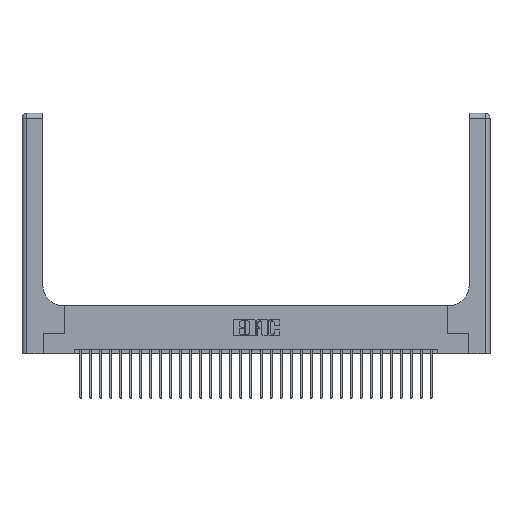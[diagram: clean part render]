
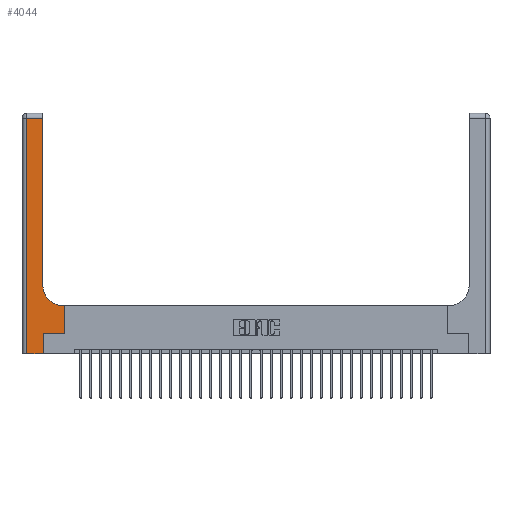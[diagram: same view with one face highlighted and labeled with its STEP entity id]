
A CAD part, top view. The second image highlights one B-rep face of the part: STEP entity #4044.
In plain terms, the highlighted planar face has unit normal (0, 0, 1).
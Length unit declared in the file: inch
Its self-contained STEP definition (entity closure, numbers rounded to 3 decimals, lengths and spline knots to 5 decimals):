
#496 = DIRECTION ( 'NONE',  ( 0., 1., 0. ) ) ;
#600 = VECTOR ( 'NONE', #2270, 39.37008 ) ;
#1074 = EDGE_CURVE ( 'NONE', #3057, #27506, #25607, .T. ) ;
#1107 = LINE ( 'NONE', #29001, #22637 ) ;
#1512 = CARTESIAN_POINT ( 'NONE',  ( 0.528, 0.6, 0.37 ) ) ;
#1595 = VERTEX_POINT ( 'NONE', #16733 ) ;
#1620 = CARTESIAN_POINT ( 'NONE',  ( 0.06, 3., 0.37 ) ) ;
#1677 = CARTESIAN_POINT ( 'NONE',  ( 0.265, 0., 0.37 ) ) ;
#1723 = DIRECTION ( 'NONE',  ( 0., 0., -1. ) ) ;
#1886 = CARTESIAN_POINT ( 'NONE',  ( 0., 3., 0.37 ) ) ;
#2270 = DIRECTION ( 'NONE',  ( 1., 0., 0. ) ) ;
#2606 = VECTOR ( 'NONE', #24935, 39.37008 ) ;
#3057 = VERTEX_POINT ( 'NONE', #15080 ) ;
#3181 = VERTEX_POINT ( 'NONE', #25020 ) ;
#3529 = CARTESIAN_POINT ( 'NONE',  ( 0.26, 0.85, 0.37 ) ) ;
#4044 = ADVANCED_FACE ( 'NONE', ( #29774 ), #22447, .F. ) ;
#4904 = ORIENTED_EDGE ( 'NONE', *, *, #13487, .T. ) ;
#5570 = CARTESIAN_POINT ( 'NONE',  ( 0.06, 2.94, 0.37 ) ) ;
#5603 = AXIS2_PLACEMENT_3D ( 'NONE', #1886, #1723, #27196 ) ;
#5758 = VECTOR ( 'NONE', #496, 39.37008 ) ;
#5967 = VERTEX_POINT ( 'NONE', #1512 ) ;
#6433 = EDGE_CURVE ( 'NONE', #5967, #1595, #26345, .T. ) ;
#7788 = ORIENTED_EDGE ( 'NONE', *, *, #6433, .T. ) ;
#7836 = CARTESIAN_POINT ( 'NONE',  ( 0., 0., 0.37 ) ) ;
#7870 = EDGE_CURVE ( 'NONE', #19559, #3181, #12021, .T. ) ;
#10801 = VERTEX_POINT ( 'NONE', #1677 ) ;
#10849 = CARTESIAN_POINT ( 'NONE',  ( 0.528, 0.25, 0.37 ) ) ;
#10912 = ORIENTED_EDGE ( 'NONE', *, *, #28871, .T. ) ;
#11046 = EDGE_CURVE ( 'NONE', #28968, #18930, #19761, .T. ) ;
#11451 = CARTESIAN_POINT ( 'NONE',  ( 0.06, 0., 0.37 ) ) ;
#11952 = ORIENTED_EDGE ( 'NONE', *, *, #7870, .T. ) ;
#12021 = LINE ( 'NONE', #23658, #5758 ) ;
#12481 = VECTOR ( 'NONE', #19462, 39.37008 ) ;
#12837 = ORIENTED_EDGE ( 'NONE', *, *, #29251, .T. ) ;
#13487 = EDGE_CURVE ( 'NONE', #10801, #3057, #1107, .T. ) ;
#14440 = EDGE_CURVE ( 'NONE', #27506, #5967, #15670, .T. ) ;
#15080 = CARTESIAN_POINT ( 'NONE',  ( 0.265, 0.25, 0.37 ) ) ;
#15579 = DIRECTION ( 'NONE',  ( 1., 0., 0. ) ) ;
#15670 = LINE ( 'NONE', #10849, #2606 ) ;
#15892 = ORIENTED_EDGE ( 'NONE', *, *, #1074, .T. ) ;
#16733 = CARTESIAN_POINT ( 'NONE',  ( 0.51, 0.6, 0.37 ) ) ;
#16999 = EDGE_LOOP ( 'NONE', ( #11952, #12837, #29147, #27119, #4904, #15892, #22238, #7788, #10912 ) ) ;
#17499 = CARTESIAN_POINT ( 'NONE',  ( 0., 2.94, 0.37 ) ) ;
#17676 = CARTESIAN_POINT ( 'NONE',  ( 0.51, 0.85, 0.37 ) ) ;
#17766 = AXIS2_PLACEMENT_3D ( 'NONE', #17676, #29094, #15579 ) ;
#18930 = VERTEX_POINT ( 'NONE', #11451 ) ;
#19005 = LINE ( 'NONE', #7836, #12481 ) ;
#19462 = DIRECTION ( 'NONE',  ( 1., 0., 0. ) ) ;
#19559 = VERTEX_POINT ( 'NONE', #3529 ) ;
#19761 = LINE ( 'NONE', #1620, #27238 ) ;
#19904 = LINE ( 'NONE', #17499, #27036 ) ;
#21795 = CARTESIAN_POINT ( 'NONE',  ( 0.528, 0.25, 0.37 ) ) ;
#22115 = VECTOR ( 'NONE', #26494, 39.37008 ) ;
#22238 = ORIENTED_EDGE ( 'NONE', *, *, #14440, .T. ) ;
#22447 = PLANE ( 'NONE',  #5603 ) ;
#22637 = VECTOR ( 'NONE', #26113, 39.37008 ) ;
#23658 = CARTESIAN_POINT ( 'NONE',  ( 0.26, 3., 0.37 ) ) ;
#24935 = DIRECTION ( 'NONE',  ( 0., 1., 0. ) ) ;
#25020 = CARTESIAN_POINT ( 'NONE',  ( 0.26, 2.94, 0.37 ) ) ;
#25607 = LINE ( 'NONE', #25903, #600 ) ;
#25903 = CARTESIAN_POINT ( 'NONE',  ( 0.265, 0.25, 0.37 ) ) ;
#26029 = CIRCLE ( 'NONE', #17766, 0.25 ) ;
#26113 = DIRECTION ( 'NONE',  ( 0., 1., 0. ) ) ;
#26188 = CARTESIAN_POINT ( 'NONE',  ( 0.26, 0.6, 0.37 ) ) ;
#26345 = LINE ( 'NONE', #26188, #22115 ) ;
#26494 = DIRECTION ( 'NONE',  ( -1., 0., 0. ) ) ;
#26788 = DIRECTION ( 'NONE',  ( -1., 0., 0. ) ) ;
#27036 = VECTOR ( 'NONE', #26788, 39.37008 ) ;
#27119 = ORIENTED_EDGE ( 'NONE', *, *, #29054, .T. ) ;
#27196 = DIRECTION ( 'NONE',  ( -1., 0., 0. ) ) ;
#27238 = VECTOR ( 'NONE', #29355, 39.37008 ) ;
#27506 = VERTEX_POINT ( 'NONE', #21795 ) ;
#28871 = EDGE_CURVE ( 'NONE', #1595, #19559, #26029, .T. ) ;
#28968 = VERTEX_POINT ( 'NONE', #5570 ) ;
#29001 = CARTESIAN_POINT ( 'NONE',  ( 0.265, 0., 0.37 ) ) ;
#29054 = EDGE_CURVE ( 'NONE', #18930, #10801, #19005, .T. ) ;
#29094 = DIRECTION ( 'NONE',  ( 0., 0., -1. ) ) ;
#29147 = ORIENTED_EDGE ( 'NONE', *, *, #11046, .T. ) ;
#29251 = EDGE_CURVE ( 'NONE', #3181, #28968, #19904, .T. ) ;
#29355 = DIRECTION ( 'NONE',  ( 0., -1., 0. ) ) ;
#29774 = FACE_OUTER_BOUND ( 'NONE', #16999, .T. ) ;
